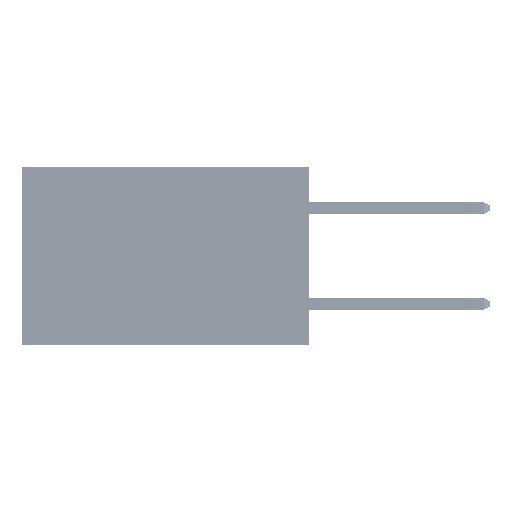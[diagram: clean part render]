
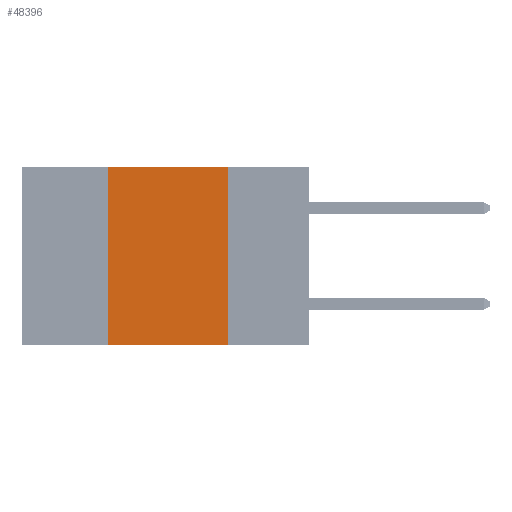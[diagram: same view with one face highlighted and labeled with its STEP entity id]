
A CAD part, left-side view. The second image highlights one B-rep face of the part: STEP entity #48396.
In plain terms, the highlighted planar face has unit normal (-1, 0, 0).
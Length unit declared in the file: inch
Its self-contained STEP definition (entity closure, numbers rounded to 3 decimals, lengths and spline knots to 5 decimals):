
#1587 = EDGE_LOOP ( 'NONE', ( #5146, #30506, #28944, #20005 ) ) ;
#5146 = ORIENTED_EDGE ( 'NONE', *, *, #12393, .F. ) ;
#5808 = VECTOR ( 'NONE', #6113, 39.37008 ) ;
#6113 = DIRECTION ( 'NONE',  ( 0., 0., -1. ) ) ;
#6338 = DIRECTION ( 'NONE',  ( 0., 0., 1. ) ) ;
#10429 = CARTESIAN_POINT ( 'NONE',  ( 0., 0.17, 0. ) ) ;
#11221 = VERTEX_POINT ( 'NONE', #10429 ) ;
#12393 = EDGE_CURVE ( 'NONE', #11221, #36185, #49234, .T. ) ;
#13285 = FACE_OUTER_BOUND ( 'NONE', #1587, .T. ) ;
#13444 = DIRECTION ( 'NONE',  ( 0., -1., 0. ) ) ;
#13722 = AXIS2_PLACEMENT_3D ( 'NONE', #18212, #37644, #41658 ) ;
#14921 = LINE ( 'NONE', #21326, #43297 ) ;
#14937 = VERTEX_POINT ( 'NONE', #19102 ) ;
#15926 = EDGE_CURVE ( 'NONE', #22671, #14937, #32837, .T. ) ;
#18212 = CARTESIAN_POINT ( 'NONE',  ( 0., 0.6, 0. ) ) ;
#19102 = CARTESIAN_POINT ( 'NONE',  ( 0., 0.42, 0. ) ) ;
#20005 = ORIENTED_EDGE ( 'NONE', *, *, #42479, .T. ) ;
#21326 = CARTESIAN_POINT ( 'NONE',  ( 0., 0.6, 0. ) ) ;
#22559 = VECTOR ( 'NONE', #6338, 39.37008 ) ;
#22671 = VERTEX_POINT ( 'NONE', #27180 ) ;
#27180 = CARTESIAN_POINT ( 'NONE',  ( 0., 0.42, -0.37 ) ) ;
#28944 = ORIENTED_EDGE ( 'NONE', *, *, #15926, .F. ) ;
#29878 = LINE ( 'NONE', #49712, #34720 ) ;
#29990 = PLANE ( 'NONE',  #13722 ) ;
#30506 = ORIENTED_EDGE ( 'NONE', *, *, #35809, .F. ) ;
#32837 = LINE ( 'NONE', #45324, #22559 ) ;
#34720 = VECTOR ( 'NONE', #41975, 39.37008 ) ;
#35809 = EDGE_CURVE ( 'NONE', #14937, #11221, #14921, .T. ) ;
#36185 = VERTEX_POINT ( 'NONE', #38903 ) ;
#37644 = DIRECTION ( 'NONE',  ( 1., 0., 0. ) ) ;
#38903 = CARTESIAN_POINT ( 'NONE',  ( 0., 0.17, -0.37 ) ) ;
#41658 = DIRECTION ( 'NONE',  ( 0., 0., -1. ) ) ;
#41975 = DIRECTION ( 'NONE',  ( 0., -1., 0. ) ) ;
#42479 = EDGE_CURVE ( 'NONE', #22671, #36185, #29878, .T. ) ;
#43297 = VECTOR ( 'NONE', #13444, 39.37008 ) ;
#45324 = CARTESIAN_POINT ( 'NONE',  ( 0., 0.42, 0. ) ) ;
#48257 = CARTESIAN_POINT ( 'NONE',  ( 0., 0.17, 0. ) ) ;
#48396 = ADVANCED_FACE ( 'NONE', ( #13285 ), #29990, .F. ) ;
#49234 = LINE ( 'NONE', #48257, #5808 ) ;
#49712 = CARTESIAN_POINT ( 'NONE',  ( 0., 0.6, -0.37 ) ) ;
